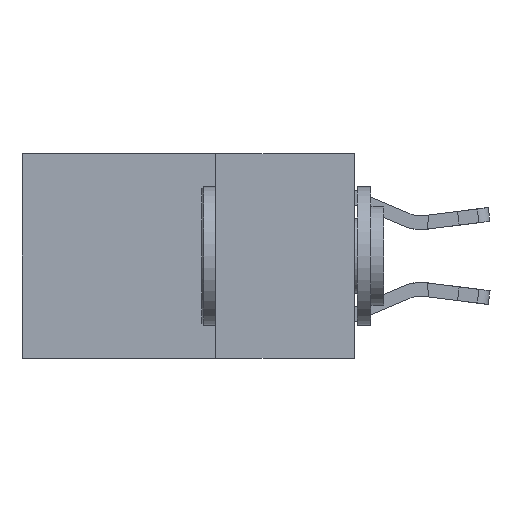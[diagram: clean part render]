
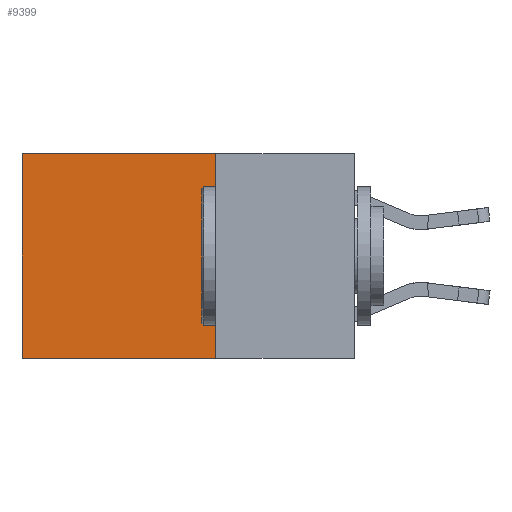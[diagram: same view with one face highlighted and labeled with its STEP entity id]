
A CAD part, left-side view. The second image highlights one B-rep face of the part: STEP entity #9399.
In plain terms, the highlighted planar face has unit normal (-1, 0, 0).
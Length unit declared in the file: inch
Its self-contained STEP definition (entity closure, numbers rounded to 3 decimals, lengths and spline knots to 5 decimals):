
#115 = DIRECTION ( 'NONE',  ( 0., 0., -1. ) ) ;
#817 = CARTESIAN_POINT ( 'NONE',  ( 0.2625, 0.25, 0. ) ) ;
#2309 = VECTOR ( 'NONE', #11648, 39.37008 ) ;
#2722 = LINE ( 'NONE', #817, #2309 ) ;
#3696 = LINE ( 'NONE', #11072, #10484 ) ;
#4191 = CARTESIAN_POINT ( 'NONE',  ( 0.2625, 0.25, -0.37 ) ) ;
#5283 = CARTESIAN_POINT ( 'NONE',  ( 0.2625, 0.25, 0. ) ) ;
#6097 = ORIENTED_EDGE ( 'NONE', *, *, #12163, .T. ) ;
#6934 = VECTOR ( 'NONE', #17462, 39.37008 ) ;
#6990 = DIRECTION ( 'NONE',  ( 0., 1., 0. ) ) ;
#7167 = CARTESIAN_POINT ( 'NONE',  ( 0.2625, 0.25, 0. ) ) ;
#8097 = ORIENTED_EDGE ( 'NONE', *, *, #11078, .F. ) ;
#8231 = DIRECTION ( 'NONE',  ( 1., 0., 0. ) ) ;
#8320 = FACE_OUTER_BOUND ( 'NONE', #15506, .T. ) ;
#8824 = CARTESIAN_POINT ( 'NONE',  ( 0.2625, 0.6, 0. ) ) ;
#9121 = LINE ( 'NONE', #8824, #11850 ) ;
#9399 = ADVANCED_FACE ( 'NONE', ( #8320 ), #16327, .F. ) ;
#9513 = CARTESIAN_POINT ( 'NONE',  ( 0.2625, 0.25, 0. ) ) ;
#10333 = CARTESIAN_POINT ( 'NONE',  ( 0.2625, 0.6, 0. ) ) ;
#10484 = VECTOR ( 'NONE', #6990, 39.37008 ) ;
#10963 = LINE ( 'NONE', #5283, #6934 ) ;
#11072 = CARTESIAN_POINT ( 'NONE',  ( 0.2625, 0.25, -0.37 ) ) ;
#11078 = EDGE_CURVE ( 'NONE', #11747, #15353, #2722, .T. ) ;
#11648 = DIRECTION ( 'NONE',  ( 0., 0., -1. ) ) ;
#11747 = VERTEX_POINT ( 'NONE', #7167 ) ;
#11850 = VECTOR ( 'NONE', #16940, 39.37008 ) ;
#12163 = EDGE_CURVE ( 'NONE', #11747, #17075, #10963, .T. ) ;
#13132 = AXIS2_PLACEMENT_3D ( 'NONE', #9513, #8231, #115 ) ;
#13406 = ORIENTED_EDGE ( 'NONE', *, *, #13560, .F. ) ;
#13421 = ORIENTED_EDGE ( 'NONE', *, *, #14970, .T. ) ;
#13560 = EDGE_CURVE ( 'NONE', #15353, #14257, #3696, .T. ) ;
#14257 = VERTEX_POINT ( 'NONE', #15175 ) ;
#14970 = EDGE_CURVE ( 'NONE', #17075, #14257, #9121, .T. ) ;
#15175 = CARTESIAN_POINT ( 'NONE',  ( 0.2625, 0.6, -0.37 ) ) ;
#15353 = VERTEX_POINT ( 'NONE', #4191 ) ;
#15506 = EDGE_LOOP ( 'NONE', ( #13421, #13406, #8097, #6097 ) ) ;
#16327 = PLANE ( 'NONE',  #13132 ) ;
#16940 = DIRECTION ( 'NONE',  ( 0., 0., -1. ) ) ;
#17075 = VERTEX_POINT ( 'NONE', #10333 ) ;
#17462 = DIRECTION ( 'NONE',  ( 0., 1., 0. ) ) ;
